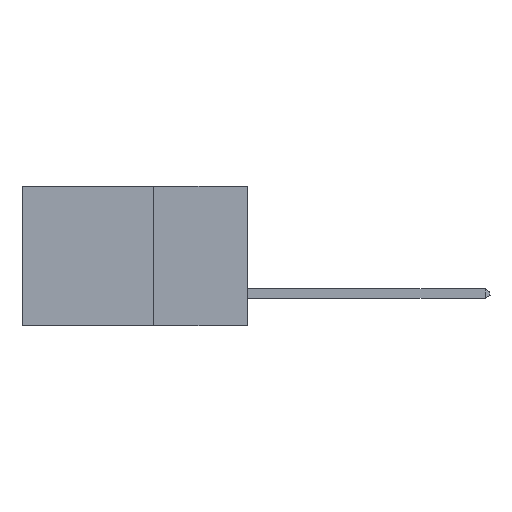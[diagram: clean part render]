
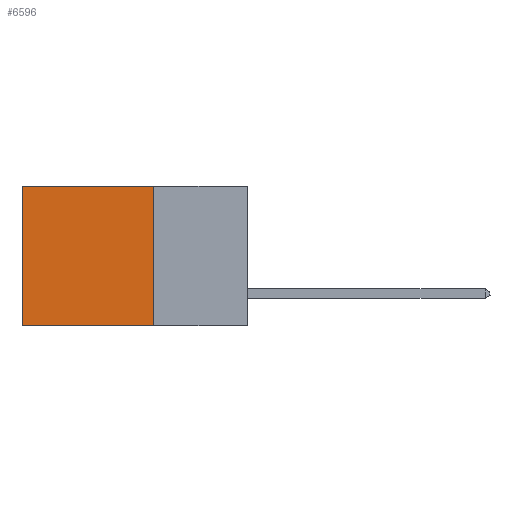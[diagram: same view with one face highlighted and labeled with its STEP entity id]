
A CAD part, left-side view. The second image highlights one B-rep face of the part: STEP entity #6596.
In plain terms, the highlighted planar face has unit normal (-1, 0, 0).
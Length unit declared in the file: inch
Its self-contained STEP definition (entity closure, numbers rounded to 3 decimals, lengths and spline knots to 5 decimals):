
#403 = VERTEX_POINT ( 'NONE', #10844 ) ;
#483 = ORIENTED_EDGE ( 'NONE', *, *, #11546, .F. ) ;
#487 = CARTESIAN_POINT ( 'NONE',  ( 0.298, 0.25, 0. ) ) ;
#715 = FACE_OUTER_BOUND ( 'NONE', #6392, .T. ) ;
#938 = EDGE_CURVE ( 'NONE', #7826, #403, #12097, .T. ) ;
#2281 = DIRECTION ( 'NONE',  ( 0., 0., -1. ) ) ;
#2479 = DIRECTION ( 'NONE',  ( 0., 0., -1. ) ) ;
#3008 = VECTOR ( 'NONE', #2281, 39.37008 ) ;
#3477 = EDGE_CURVE ( 'NONE', #8078, #8231, #9723, .T. ) ;
#3780 = CARTESIAN_POINT ( 'NONE',  ( 0.298, 0.6, 0. ) ) ;
#4118 = ORIENTED_EDGE ( 'NONE', *, *, #4326, .T. ) ;
#4326 = EDGE_CURVE ( 'NONE', #7826, #8078, #5370, .T. ) ;
#4379 = DIRECTION ( 'NONE',  ( 0., 1., 0. ) ) ;
#4728 = DIRECTION ( 'NONE',  ( 0., 0., -1. ) ) ;
#5370 = LINE ( 'NONE', #6787, #12313 ) ;
#5696 = LINE ( 'NONE', #9223, #10626 ) ;
#6190 = CARTESIAN_POINT ( 'NONE',  ( 0.298, 0.25, 0. ) ) ;
#6217 = CARTESIAN_POINT ( 'NONE',  ( 0.298, 0.6, -0.37 ) ) ;
#6392 = EDGE_LOOP ( 'NONE', ( #9686, #483, #6920, #4118 ) ) ;
#6596 = ADVANCED_FACE ( 'NONE', ( #715 ), #12225, .F. ) ;
#6787 = CARTESIAN_POINT ( 'NONE',  ( 0.298, 0.25, 0. ) ) ;
#6920 = ORIENTED_EDGE ( 'NONE', *, *, #938, .F. ) ;
#7557 = CARTESIAN_POINT ( 'NONE',  ( 0.298, 0.25, 0. ) ) ;
#7826 = VERTEX_POINT ( 'NONE', #7557 ) ;
#8078 = VERTEX_POINT ( 'NONE', #10930 ) ;
#8231 = VERTEX_POINT ( 'NONE', #6217 ) ;
#8401 = DIRECTION ( 'NONE',  ( 1., 0., 0. ) ) ;
#9223 = CARTESIAN_POINT ( 'NONE',  ( 0.298, 0.25, -0.37 ) ) ;
#9406 = VECTOR ( 'NONE', #4728, 39.37008 ) ;
#9686 = ORIENTED_EDGE ( 'NONE', *, *, #3477, .T. ) ;
#9723 = LINE ( 'NONE', #3780, #9406 ) ;
#9778 = DIRECTION ( 'NONE',  ( 0., 1., 0. ) ) ;
#10626 = VECTOR ( 'NONE', #4379, 39.37008 ) ;
#10844 = CARTESIAN_POINT ( 'NONE',  ( 0.298, 0.25, -0.37 ) ) ;
#10930 = CARTESIAN_POINT ( 'NONE',  ( 0.298, 0.6, 0. ) ) ;
#11546 = EDGE_CURVE ( 'NONE', #403, #8231, #5696, .T. ) ;
#11696 = AXIS2_PLACEMENT_3D ( 'NONE', #487, #8401, #2479 ) ;
#12097 = LINE ( 'NONE', #6190, #3008 ) ;
#12225 = PLANE ( 'NONE',  #11696 ) ;
#12313 = VECTOR ( 'NONE', #9778, 39.37008 ) ;
